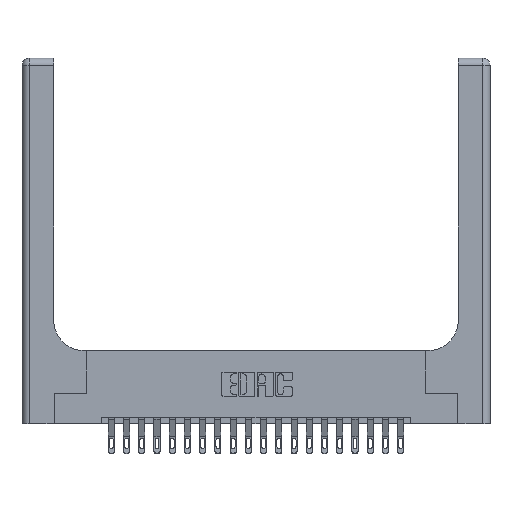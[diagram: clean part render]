
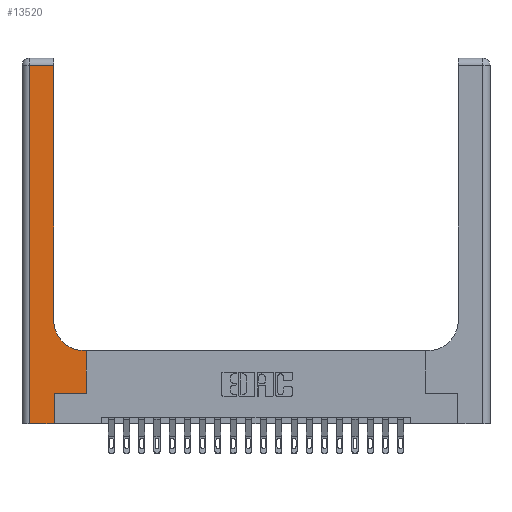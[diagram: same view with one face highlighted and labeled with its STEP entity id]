
A CAD part, top view. The second image highlights one B-rep face of the part: STEP entity #13520.
In plain terms, the highlighted planar face has unit normal (0, 0, 1).
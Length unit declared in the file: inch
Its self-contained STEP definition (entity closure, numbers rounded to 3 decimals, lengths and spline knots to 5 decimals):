
#758 = VECTOR ( 'NONE', #18213, 39.37008 ) ;
#1397 = ORIENTED_EDGE ( 'NONE', *, *, #20136, .T. ) ;
#1721 = CARTESIAN_POINT ( 'NONE',  ( 0.528, 0.25, 0.37 ) ) ;
#1732 = LINE ( 'NONE', #17480, #5174 ) ;
#1819 = ORIENTED_EDGE ( 'NONE', *, *, #10560, .T. ) ;
#1821 = VECTOR ( 'NONE', #4421, 39.37008 ) ;
#1967 = ORIENTED_EDGE ( 'NONE', *, *, #17147, .T. ) ;
#2163 = CARTESIAN_POINT ( 'NONE',  ( 0.06, 3., 0.37 ) ) ;
#2417 = LINE ( 'NONE', #20775, #19033 ) ;
#2671 = LINE ( 'NONE', #5724, #9923 ) ;
#2713 = ORIENTED_EDGE ( 'NONE', *, *, #16514, .T. ) ;
#2890 = DIRECTION ( 'NONE',  ( 0., 0., -1. ) ) ;
#3119 = CARTESIAN_POINT ( 'NONE',  ( 0.265, 0.25, 0.37 ) ) ;
#3454 = LINE ( 'NONE', #12203, #3974 ) ;
#3666 = DIRECTION ( 'NONE',  ( 0., 0., -1. ) ) ;
#3974 = VECTOR ( 'NONE', #17172, 39.37008 ) ;
#4119 = EDGE_CURVE ( 'NONE', #5811, #5830, #17541, .T. ) ;
#4336 = LINE ( 'NONE', #2163, #5924 ) ;
#4421 = DIRECTION ( 'NONE',  ( 1., 0., 0. ) ) ;
#5174 = VECTOR ( 'NONE', #12793, 39.37008 ) ;
#5395 = CARTESIAN_POINT ( 'NONE',  ( 0., 0., 0.37 ) ) ;
#5524 = DIRECTION ( 'NONE',  ( 0., 1., 0. ) ) ;
#5724 = CARTESIAN_POINT ( 'NONE',  ( 0.265, 0., 0.37 ) ) ;
#5734 = VERTEX_POINT ( 'NONE', #20900 ) ;
#5759 = CARTESIAN_POINT ( 'NONE',  ( 0.06, 0., 0.37 ) ) ;
#5811 = VERTEX_POINT ( 'NONE', #16182 ) ;
#5830 = VERTEX_POINT ( 'NONE', #14648 ) ;
#5924 = VECTOR ( 'NONE', #11976, 39.37008 ) ;
#6110 = ORIENTED_EDGE ( 'NONE', *, *, #19797, .T. ) ;
#6270 = EDGE_CURVE ( 'NONE', #9155, #5811, #2417, .T. ) ;
#6731 = VERTEX_POINT ( 'NONE', #5759 ) ;
#7435 = VERTEX_POINT ( 'NONE', #17648 ) ;
#8097 = EDGE_CURVE ( 'NONE', #7435, #9155, #9934, .T. ) ;
#9155 = VERTEX_POINT ( 'NONE', #14720 ) ;
#9257 = CARTESIAN_POINT ( 'NONE',  ( 0.265, 0.25, 0.37 ) ) ;
#9771 = VERTEX_POINT ( 'NONE', #11522 ) ;
#9923 = VECTOR ( 'NONE', #5524, 39.37008 ) ;
#9934 = LINE ( 'NONE', #1721, #758 ) ;
#10560 = EDGE_CURVE ( 'NONE', #6731, #15621, #13286, .T. ) ;
#10833 = DIRECTION ( 'NONE',  ( -1., 0., 0. ) ) ;
#10976 = EDGE_CURVE ( 'NONE', #11663, #7435, #17389, .T. ) ;
#11126 = AXIS2_PLACEMENT_3D ( 'NONE', #20176, #3666, #17373 ) ;
#11522 = CARTESIAN_POINT ( 'NONE',  ( 0.06, 2.94, 0.37 ) ) ;
#11663 = VERTEX_POINT ( 'NONE', #9257 ) ;
#11976 = DIRECTION ( 'NONE',  ( 0., -1., 0. ) ) ;
#12203 = CARTESIAN_POINT ( 'NONE',  ( 0.26, 3., 0.37 ) ) ;
#12681 = FACE_OUTER_BOUND ( 'NONE', #13055, .T. ) ;
#12793 = DIRECTION ( 'NONE',  ( -1., 0., 0. ) ) ;
#13055 = EDGE_LOOP ( 'NONE', ( #1967, #6110, #1397, #1819, #2713, #14481, #18858, #17210, #15239 ) ) ;
#13286 = LINE ( 'NONE', #5395, #20026 ) ;
#13520 = ADVANCED_FACE ( 'NONE', ( #12681 ), #17673, .F. ) ;
#13888 = CARTESIAN_POINT ( 'NONE',  ( 0.265, 0., 0.37 ) ) ;
#14481 = ORIENTED_EDGE ( 'NONE', *, *, #10976, .T. ) ;
#14648 = CARTESIAN_POINT ( 'NONE',  ( 0.26, 0.85, 0.37 ) ) ;
#14720 = CARTESIAN_POINT ( 'NONE',  ( 0.528, 0.6, 0.37 ) ) ;
#15239 = ORIENTED_EDGE ( 'NONE', *, *, #4119, .T. ) ;
#15621 = VERTEX_POINT ( 'NONE', #13888 ) ;
#16182 = CARTESIAN_POINT ( 'NONE',  ( 0.51, 0.6, 0.37 ) ) ;
#16514 = EDGE_CURVE ( 'NONE', #15621, #11663, #2671, .T. ) ;
#16865 = DIRECTION ( 'NONE',  ( 1., 0., 0. ) ) ;
#17147 = EDGE_CURVE ( 'NONE', #5830, #5734, #3454, .T. ) ;
#17172 = DIRECTION ( 'NONE',  ( 0., 1., 0. ) ) ;
#17210 = ORIENTED_EDGE ( 'NONE', *, *, #6270, .T. ) ;
#17373 = DIRECTION ( 'NONE',  ( 1., 0., 0. ) ) ;
#17389 = LINE ( 'NONE', #3119, #1821 ) ;
#17480 = CARTESIAN_POINT ( 'NONE',  ( 0., 2.94, 0.37 ) ) ;
#17541 = CIRCLE ( 'NONE', #11126, 0.25 ) ;
#17648 = CARTESIAN_POINT ( 'NONE',  ( 0.528, 0.25, 0.37 ) ) ;
#17673 = PLANE ( 'NONE',  #18468 ) ;
#18213 = DIRECTION ( 'NONE',  ( 0., 1., 0. ) ) ;
#18468 = AXIS2_PLACEMENT_3D ( 'NONE', #19629, #2890, #19562 ) ;
#18858 = ORIENTED_EDGE ( 'NONE', *, *, #8097, .T. ) ;
#19033 = VECTOR ( 'NONE', #10833, 39.37008 ) ;
#19562 = DIRECTION ( 'NONE',  ( -1., 0., 0. ) ) ;
#19629 = CARTESIAN_POINT ( 'NONE',  ( 0., 3., 0.37 ) ) ;
#19797 = EDGE_CURVE ( 'NONE', #5734, #9771, #1732, .T. ) ;
#20026 = VECTOR ( 'NONE', #16865, 39.37008 ) ;
#20136 = EDGE_CURVE ( 'NONE', #9771, #6731, #4336, .T. ) ;
#20176 = CARTESIAN_POINT ( 'NONE',  ( 0.51, 0.85, 0.37 ) ) ;
#20775 = CARTESIAN_POINT ( 'NONE',  ( 0.26, 0.6, 0.37 ) ) ;
#20900 = CARTESIAN_POINT ( 'NONE',  ( 0.26, 2.94, 0.37 ) ) ;
